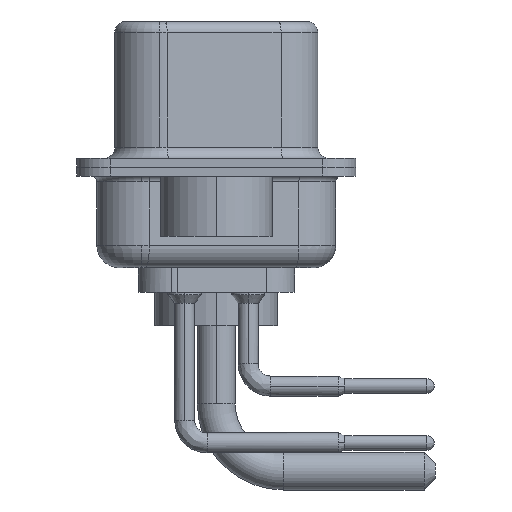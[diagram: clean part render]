
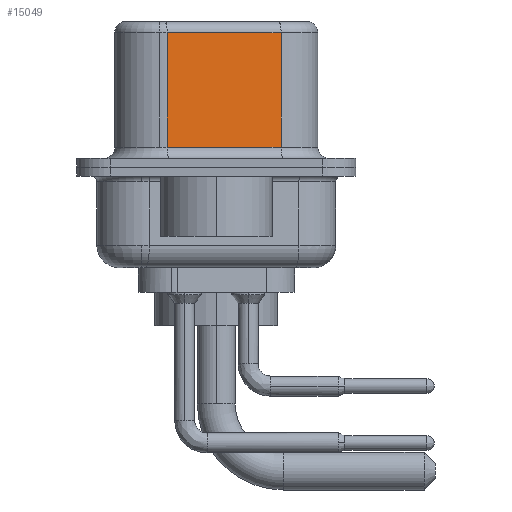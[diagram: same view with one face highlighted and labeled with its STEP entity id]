
A CAD part, left-side view. The second image highlights one B-rep face of the part: STEP entity #15049.
In plain terms, the highlighted planar face has unit normal (-0.985, -0.174, 0).
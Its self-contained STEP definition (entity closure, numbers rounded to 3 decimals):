
#652 = DIRECTION ( 'NONE',  ( 0.985, 0.174, 0. ) ) ;
#874 = EDGE_CURVE ( 'NONE', #25230, #12052, #10758, .T. ) ;
#2140 = AXIS2_PLACEMENT_3D ( 'NONE', #2639, #652, #20069 ) ;
#2372 = ORIENTED_EDGE ( 'NONE', *, *, #3470, .F. ) ;
#2639 = CARTESIAN_POINT ( 'NONE',  ( 4.58, -2.897, 6.52 ) ) ;
#3379 = LINE ( 'NONE', #25650, #20899 ) ;
#3470 = EDGE_CURVE ( 'NONE', #7487, #11097, #19710, .T. ) ;
#4374 = ORIENTED_EDGE ( 'NONE', *, *, #19503, .T. ) ;
#5672 = DIRECTION ( 'NONE',  ( 0.174, -0.985, 0. ) ) ;
#6313 = FACE_OUTER_BOUND ( 'NONE', #6758, .T. ) ;
#6758 = EDGE_LOOP ( 'NONE', ( #2372, #7866, #19275, #4374 ) ) ;
#7487 = VERTEX_POINT ( 'NONE', #17944 ) ;
#7866 = ORIENTED_EDGE ( 'NONE', *, *, #13887, .T. ) ;
#10630 = CARTESIAN_POINT ( 'NONE',  ( 3.68, 2.203, 6.52 ) ) ;
#10758 = LINE ( 'NONE', #10630, #14230 ) ;
#11097 = VERTEX_POINT ( 'NONE', #25509 ) ;
#12052 = VERTEX_POINT ( 'NONE', #14931 ) ;
#13887 = EDGE_CURVE ( 'NONE', #7487, #25230, #3379, .T. ) ;
#14230 = VECTOR ( 'NONE', #24654, 1000. ) ;
#14931 = CARTESIAN_POINT ( 'NONE',  ( 3.68, 2.203, 0.9 ) ) ;
#15049 = ADVANCED_FACE ( 'NONE', ( #6313 ), #22029, .F. ) ;
#16425 = CARTESIAN_POINT ( 'NONE',  ( 3.68, 2.203, 6.02 ) ) ;
#17944 = CARTESIAN_POINT ( 'NONE',  ( 4.58, -2.897, 6.02 ) ) ;
#18055 = DIRECTION ( 'NONE',  ( -0.174, 0.985, 0. ) ) ;
#18589 = VECTOR ( 'NONE', #5672, 1000. ) ;
#19275 = ORIENTED_EDGE ( 'NONE', *, *, #874, .T. ) ;
#19503 = EDGE_CURVE ( 'NONE', #12052, #11097, #21412, .T. ) ;
#19710 = LINE ( 'NONE', #23405, #21103 ) ;
#20069 = DIRECTION ( 'NONE',  ( -0.174, 0.985, 0. ) ) ;
#20899 = VECTOR ( 'NONE', #18055, 1000. ) ;
#21103 = VECTOR ( 'NONE', #21553, 1000. ) ;
#21412 = LINE ( 'NONE', #23121, #18589 ) ;
#21553 = DIRECTION ( 'NONE',  ( 0., 0., -1. ) ) ;
#22029 = PLANE ( 'NONE',  #2140 ) ;
#23121 = CARTESIAN_POINT ( 'NONE',  ( 4.58, -2.897, 0.9 ) ) ;
#23405 = CARTESIAN_POINT ( 'NONE',  ( 4.58, -2.897, 6.52 ) ) ;
#24654 = DIRECTION ( 'NONE',  ( 0., 0., -1. ) ) ;
#25230 = VERTEX_POINT ( 'NONE', #16425 ) ;
#25509 = CARTESIAN_POINT ( 'NONE',  ( 4.58, -2.897, 0.9 ) ) ;
#25650 = CARTESIAN_POINT ( 'NONE',  ( 4.58, -2.897, 6.02 ) ) ;
